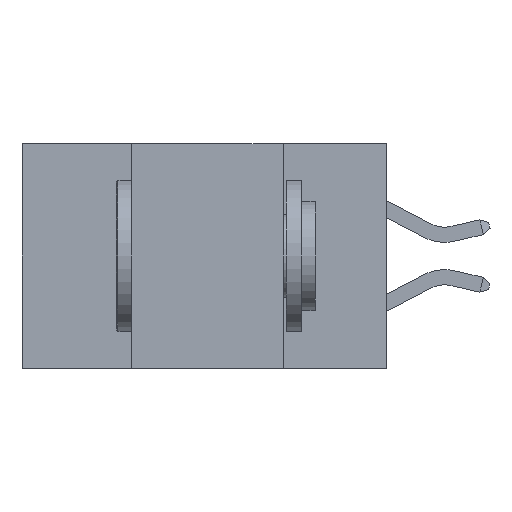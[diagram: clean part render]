
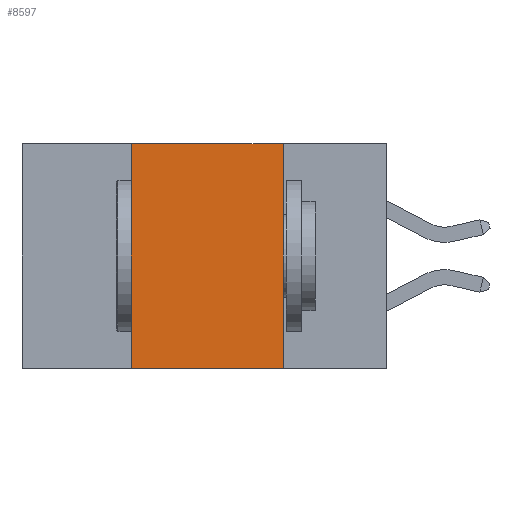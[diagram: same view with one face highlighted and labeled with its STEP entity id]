
A CAD part, left-side view. The second image highlights one B-rep face of the part: STEP entity #8597.
In plain terms, the highlighted planar face has unit normal (-1, 0, 0).
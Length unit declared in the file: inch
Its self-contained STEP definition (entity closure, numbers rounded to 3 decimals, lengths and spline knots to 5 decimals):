
#1326 = CARTESIAN_POINT ( 'NONE',  ( 0., 0.6, 0. ) ) ;
#2070 = CARTESIAN_POINT ( 'NONE',  ( 0., 0.6, -0.37 ) ) ;
#2624 = VECTOR ( 'NONE', #13638, 39.37008 ) ;
#3457 = CARTESIAN_POINT ( 'NONE',  ( 0., 0.42, 0. ) ) ;
#3708 = AXIS2_PLACEMENT_3D ( 'NONE', #1326, #21262, #28986 ) ;
#4706 = DIRECTION ( 'NONE',  ( 0., 0., 1. ) ) ;
#6343 = PLANE ( 'NONE',  #3708 ) ;
#6966 = DIRECTION ( 'NONE',  ( 0., -1., 0. ) ) ;
#7860 = DIRECTION ( 'NONE',  ( 0., 0., -1. ) ) ;
#8597 = ADVANCED_FACE ( 'NONE', ( #10192 ), #6343, .F. ) ;
#9052 = CARTESIAN_POINT ( 'NONE',  ( 0., 0.6, 0. ) ) ;
#9256 = LINE ( 'NONE', #9052, #2624 ) ;
#10192 = FACE_OUTER_BOUND ( 'NONE', #14669, .T. ) ;
#10212 = LINE ( 'NONE', #29864, #32083 ) ;
#11334 = VERTEX_POINT ( 'NONE', #15630 ) ;
#13638 = DIRECTION ( 'NONE',  ( 0., -1., 0. ) ) ;
#14669 = EDGE_LOOP ( 'NONE', ( #32036, #26839, #28666, #27477 ) ) ;
#14831 = EDGE_CURVE ( 'NONE', #19616, #11334, #10212, .T. ) ;
#15630 = CARTESIAN_POINT ( 'NONE',  ( 0., 0.17, -0.37 ) ) ;
#16494 = CARTESIAN_POINT ( 'NONE',  ( 0., 0.42, -0.37 ) ) ;
#16903 = CARTESIAN_POINT ( 'NONE',  ( 0., 0.17, 0. ) ) ;
#17365 = EDGE_CURVE ( 'NONE', #17798, #19616, #9256, .T. ) ;
#17798 = VERTEX_POINT ( 'NONE', #3457 ) ;
#18479 = VERTEX_POINT ( 'NONE', #16494 ) ;
#18723 = EDGE_CURVE ( 'NONE', #18479, #17798, #27130, .T. ) ;
#19028 = LINE ( 'NONE', #2070, #19396 ) ;
#19396 = VECTOR ( 'NONE', #6966, 39.37008 ) ;
#19616 = VERTEX_POINT ( 'NONE', #16903 ) ;
#19743 = CARTESIAN_POINT ( 'NONE',  ( 0., 0.42, 0. ) ) ;
#21262 = DIRECTION ( 'NONE',  ( 1., 0., 0. ) ) ;
#21376 = EDGE_CURVE ( 'NONE', #18479, #11334, #19028, .T. ) ;
#23224 = VECTOR ( 'NONE', #4706, 39.37008 ) ;
#26839 = ORIENTED_EDGE ( 'NONE', *, *, #17365, .F. ) ;
#27130 = LINE ( 'NONE', #19743, #23224 ) ;
#27477 = ORIENTED_EDGE ( 'NONE', *, *, #21376, .T. ) ;
#28666 = ORIENTED_EDGE ( 'NONE', *, *, #18723, .F. ) ;
#28986 = DIRECTION ( 'NONE',  ( 0., 0., -1. ) ) ;
#29864 = CARTESIAN_POINT ( 'NONE',  ( 0., 0.17, 0. ) ) ;
#32036 = ORIENTED_EDGE ( 'NONE', *, *, #14831, .F. ) ;
#32083 = VECTOR ( 'NONE', #7860, 39.37008 ) ;
